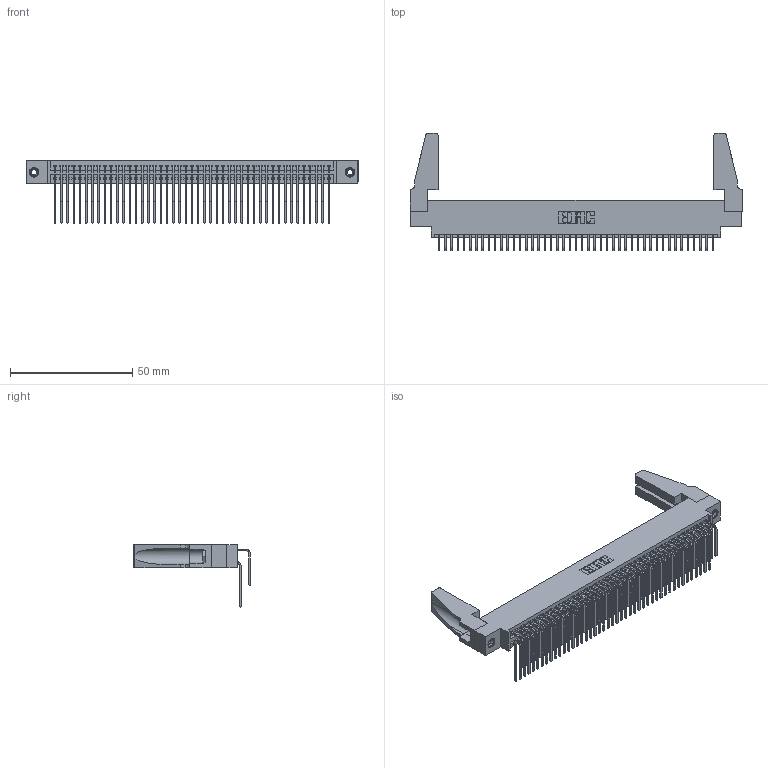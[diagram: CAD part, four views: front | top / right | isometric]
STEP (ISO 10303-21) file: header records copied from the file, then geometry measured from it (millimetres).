
FILE_DESCRIPTION (( 'STEP AP203' ), '1' );
FILE_NAME ('395-090-559-888.STEP', '2019-10-25T18:07:18', ( '' ), ( '' ), 'SwSTEP 2.0', 'SolidWorks 2016', '' );
FILE_SCHEMA (( 'CONFIG_CONTROL_DESIGN' ));
Length unit declared in the file: inch
Products named in the file (6): 395-090-559-888; 345 Part_0.170 Offset - 0.156 Dia-TH; 345-292-001_558 559 Tail - 1; 345-292-001_559 Tail - 2; 345-250-001_345-250-001-102; 345-220-078_345-220-088
Assembly tree (95 placements, depth 2):
  395-090-559-888
    345 Part_0.170 Offset - 0.156 Dia-TH
    345-292-001_558 559 Tail - 1  x45
    345-292-001_559 Tail - 2  x45
    345-250-001_345-250-001-102  x2
    345-220-078_345-220-088  x2
Bounding box: 135.53 x 47.74 x 25.53 mm (x, y, z)
Volume: 16852 mm3; surface area: 25867.6 mm2
Topology: 95 solids, 95 shells, 4934 faces, 14617 edges, 9614 vertices
Faces by surface type: plane 3306, cylinder 1612, cone 12, torus 4
Entity records: 38836 total; most frequent: CARTESIAN_POINT 6549, ORIENTED_EDGE 6392, DIRECTION 5748, EDGE_CURVE 3196, VECTOR 2802, LINE 2802, VERTEX_POINT 2122, AXIS2_PLACEMENT_3D 1473
